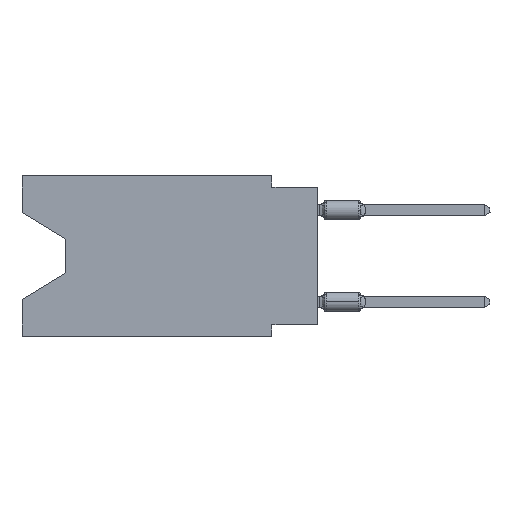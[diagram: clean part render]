
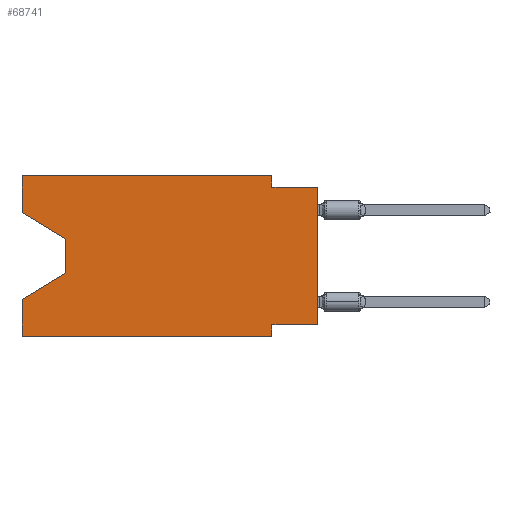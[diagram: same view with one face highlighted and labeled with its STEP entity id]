
A CAD part, left-side view. The second image highlights one B-rep face of the part: STEP entity #68741.
In plain terms, the highlighted planar face has unit normal (-1, 0, 0).
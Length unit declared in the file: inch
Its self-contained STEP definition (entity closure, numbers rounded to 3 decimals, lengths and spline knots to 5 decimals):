
#836 = ORIENTED_EDGE ( 'NONE', *, *, #19082, .T. ) ;
#1195 = DIRECTION ( 'NONE',  ( 0., 0., 1. ) ) ;
#2584 = VERTEX_POINT ( 'NONE', #40707 ) ;
#5761 = CARTESIAN_POINT ( 'NONE',  ( 0., 0.55, -0.138 ) ) ;
#7295 = VERTEX_POINT ( 'NONE', #64860 ) ;
#9634 = CARTESIAN_POINT ( 'NONE',  ( 0., 0.645, 0. ) ) ;
#9683 = DIRECTION ( 'NONE',  ( 1., 0., 0. ) ) ;
#11515 = CARTESIAN_POINT ( 'NONE',  ( 0., 0.645, -0.26975 ) ) ;
#14175 = LINE ( 'NONE', #25327, #35127 ) ;
#14422 = ORIENTED_EDGE ( 'NONE', *, *, #20751, .F. ) ;
#14771 = VECTOR ( 'NONE', #22794, 39.37008 ) ;
#15669 = VECTOR ( 'NONE', #45948, 39.37008 ) ;
#16247 = DIRECTION ( 'NONE',  ( 0., -1., 0. ) ) ;
#16654 = VERTEX_POINT ( 'NONE', #64314 ) ;
#16872 = CARTESIAN_POINT ( 'NONE',  ( 0., 0.645, 0. ) ) ;
#16901 = AXIS2_PLACEMENT_3D ( 'NONE', #65949, #9683, #43955 ) ;
#17590 = CARTESIAN_POINT ( 'NONE',  ( 0., 0.645, 0. ) ) ;
#18059 = VECTOR ( 'NONE', #32388, 39.37008 ) ;
#18123 = LINE ( 'NONE', #23365, #67038 ) ;
#19082 = EDGE_CURVE ( 'NONE', #71422, #7295, #33683, .T. ) ;
#19379 = VECTOR ( 'NONE', #65128, 39.37008 ) ;
#20751 = EDGE_CURVE ( 'NONE', #16654, #56417, #53213, .T. ) ;
#21421 = EDGE_CURVE ( 'NONE', #47240, #29023, #51861, .T. ) ;
#22132 = DIRECTION ( 'NONE',  ( 0., 0.855, -0.519 ) ) ;
#22794 = DIRECTION ( 'NONE',  ( 0., 0., 1. ) ) ;
#22952 = ORIENTED_EDGE ( 'NONE', *, *, #43237, .F. ) ;
#23365 = CARTESIAN_POINT ( 'NONE',  ( 0., 0.1, 0. ) ) ;
#24045 = VERTEX_POINT ( 'NONE', #64823 ) ;
#24107 = VECTOR ( 'NONE', #72239, 39.37008 ) ;
#25327 = CARTESIAN_POINT ( 'NONE',  ( 0., 0.645, -0.08025 ) ) ;
#25946 = ORIENTED_EDGE ( 'NONE', *, *, #53072, .F. ) ;
#26488 = EDGE_CURVE ( 'NONE', #58336, #43259, #18123, .T. ) ;
#27425 = LINE ( 'NONE', #51259, #59159 ) ;
#28115 = DIRECTION ( 'NONE',  ( 0., 0., -1. ) ) ;
#29023 = VERTEX_POINT ( 'NONE', #11515 ) ;
#29781 = CARTESIAN_POINT ( 'NONE',  ( 0., 0.645, -0.35 ) ) ;
#29984 = EDGE_CURVE ( 'NONE', #24045, #71422, #14175, .T. ) ;
#30815 = ORIENTED_EDGE ( 'NONE', *, *, #21421, .F. ) ;
#31131 = VECTOR ( 'NONE', #28115, 39.37008 ) ;
#31160 = ORIENTED_EDGE ( 'NONE', *, *, #26488, .F. ) ;
#32388 = DIRECTION ( 'NONE',  ( 0., 0., -1. ) ) ;
#32612 = LINE ( 'NONE', #42713, #35811 ) ;
#33683 = LINE ( 'NONE', #5761, #31131 ) ;
#35105 = CARTESIAN_POINT ( 'NONE',  ( 0., 0.1, -0.025 ) ) ;
#35127 = VECTOR ( 'NONE', #49172, 39.37008 ) ;
#35811 = VECTOR ( 'NONE', #54257, 39.37008 ) ;
#37322 = ORIENTED_EDGE ( 'NONE', *, *, #40754, .T. ) ;
#40502 = DIRECTION ( 'NONE',  ( 0., 0., -1. ) ) ;
#40707 = CARTESIAN_POINT ( 'NONE',  ( 0., 0.1, -0.35 ) ) ;
#40754 = EDGE_CURVE ( 'NONE', #47240, #2584, #27425, .T. ) ;
#42660 = CARTESIAN_POINT ( 'NONE',  ( 0., 0.1, -0.325 ) ) ;
#42713 = CARTESIAN_POINT ( 'NONE',  ( 0., 0., -0.025 ) ) ;
#42853 = LINE ( 'NONE', #59995, #18059 ) ;
#43237 = EDGE_CURVE ( 'NONE', #24045, #48790, #63075, .T. ) ;
#43259 = VERTEX_POINT ( 'NONE', #35105 ) ;
#43955 = DIRECTION ( 'NONE',  ( 0., 0., -1. ) ) ;
#45928 = CARTESIAN_POINT ( 'NONE',  ( 0., 0.55, -0.138 ) ) ;
#45948 = DIRECTION ( 'NONE',  ( 0., 0., 1. ) ) ;
#47240 = VERTEX_POINT ( 'NONE', #29781 ) ;
#48456 = ORIENTED_EDGE ( 'NONE', *, *, #68775, .F. ) ;
#48790 = VERTEX_POINT ( 'NONE', #52332 ) ;
#49172 = DIRECTION ( 'NONE',  ( 0., -0.855, -0.519 ) ) ;
#49305 = EDGE_CURVE ( 'NONE', #48790, #58336, #60693, .T. ) ;
#51259 = CARTESIAN_POINT ( 'NONE',  ( 0., 0.645, -0.35 ) ) ;
#51713 = ORIENTED_EDGE ( 'NONE', *, *, #49305, .F. ) ;
#51861 = LINE ( 'NONE', #17590, #14771 ) ;
#52332 = CARTESIAN_POINT ( 'NONE',  ( 0., 0.645, 0. ) ) ;
#52716 = ORIENTED_EDGE ( 'NONE', *, *, #53661, .T. ) ;
#53072 = EDGE_CURVE ( 'NONE', #43259, #56477, #32612, .T. ) ;
#53213 = LINE ( 'NONE', #58433, #19379 ) ;
#53661 = EDGE_CURVE ( 'NONE', #16654, #56477, #69766, .T. ) ;
#54257 = DIRECTION ( 'NONE',  ( 0., -1., 0. ) ) ;
#54992 = EDGE_LOOP ( 'NONE', ( #64626, #836, #69162, #30815, #37322, #48456, #14422, #52716, #25946, #31160, #51713, #22952 ) ) ;
#56412 = VECTOR ( 'NONE', #22132, 39.37008 ) ;
#56417 = VERTEX_POINT ( 'NONE', #42660 ) ;
#56477 = VERTEX_POINT ( 'NONE', #58337 ) ;
#56548 = EDGE_CURVE ( 'NONE', #7295, #29023, #60548, .T. ) ;
#58336 = VERTEX_POINT ( 'NONE', #68627 ) ;
#58337 = CARTESIAN_POINT ( 'NONE',  ( 0., 0., -0.025 ) ) ;
#58433 = CARTESIAN_POINT ( 'NONE',  ( 0., 0., -0.325 ) ) ;
#59159 = VECTOR ( 'NONE', #16247, 39.37008 ) ;
#59626 = PLANE ( 'NONE',  #16901 ) ;
#59995 = CARTESIAN_POINT ( 'NONE',  ( 0., 0.1, -0.35 ) ) ;
#60548 = LINE ( 'NONE', #72464, #56412 ) ;
#60693 = LINE ( 'NONE', #9634, #24107 ) ;
#60735 = FACE_OUTER_BOUND ( 'NONE', #54992, .T. ) ;
#63075 = LINE ( 'NONE', #16872, #65323 ) ;
#64175 = CARTESIAN_POINT ( 'NONE',  ( 0., 0., 0. ) ) ;
#64314 = CARTESIAN_POINT ( 'NONE',  ( 0., 0., -0.325 ) ) ;
#64626 = ORIENTED_EDGE ( 'NONE', *, *, #29984, .T. ) ;
#64823 = CARTESIAN_POINT ( 'NONE',  ( 0., 0.645, -0.08025 ) ) ;
#64860 = CARTESIAN_POINT ( 'NONE',  ( 0., 0.55, -0.212 ) ) ;
#65128 = DIRECTION ( 'NONE',  ( 0., 1., 0. ) ) ;
#65323 = VECTOR ( 'NONE', #1195, 39.37008 ) ;
#65949 = CARTESIAN_POINT ( 'NONE',  ( 0., 0.645, 0. ) ) ;
#67038 = VECTOR ( 'NONE', #40502, 39.37008 ) ;
#68627 = CARTESIAN_POINT ( 'NONE',  ( 0., 0.1, 0. ) ) ;
#68741 = ADVANCED_FACE ( 'NONE', ( #60735 ), #59626, .F. ) ;
#68775 = EDGE_CURVE ( 'NONE', #56417, #2584, #42853, .T. ) ;
#69162 = ORIENTED_EDGE ( 'NONE', *, *, #56548, .T. ) ;
#69766 = LINE ( 'NONE', #64175, #15669 ) ;
#71422 = VERTEX_POINT ( 'NONE', #45928 ) ;
#72239 = DIRECTION ( 'NONE',  ( 0., -1., 0. ) ) ;
#72464 = CARTESIAN_POINT ( 'NONE',  ( 0., 0.55, -0.212 ) ) ;
